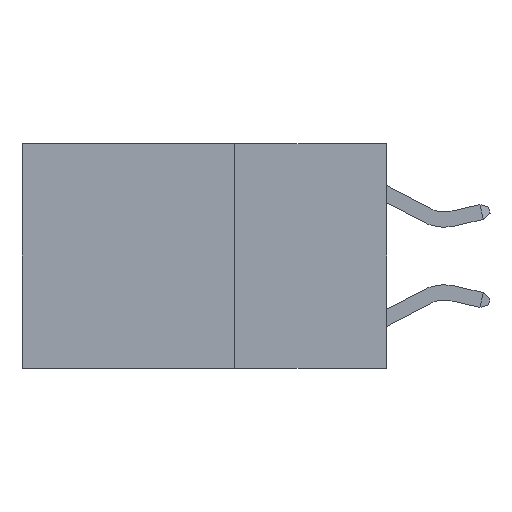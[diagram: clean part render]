
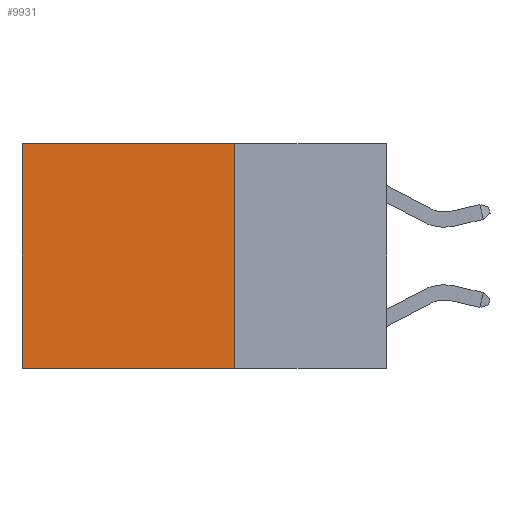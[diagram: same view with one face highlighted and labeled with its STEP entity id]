
A CAD part, left-side view. The second image highlights one B-rep face of the part: STEP entity #9931.
In plain terms, the highlighted planar face has unit normal (-1, 0, 0).
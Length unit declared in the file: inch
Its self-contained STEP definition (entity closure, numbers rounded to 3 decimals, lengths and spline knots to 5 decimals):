
#650 = VERTEX_POINT ( 'NONE', #3282 ) ;
#658 = CARTESIAN_POINT ( 'NONE',  ( 0.2625, 0.25, 0. ) ) ;
#1146 = CARTESIAN_POINT ( 'NONE',  ( 0.2625, 0.6, 0. ) ) ;
#1256 = VECTOR ( 'NONE', #19972, 39.37008 ) ;
#2601 = ORIENTED_EDGE ( 'NONE', *, *, #5508, .F. ) ;
#3282 = CARTESIAN_POINT ( 'NONE',  ( 0.2625, 0.25, 0. ) ) ;
#3354 = VERTEX_POINT ( 'NONE', #8231 ) ;
#3505 = LINE ( 'NONE', #1146, #19360 ) ;
#4098 = VERTEX_POINT ( 'NONE', #19634 ) ;
#4163 = LINE ( 'NONE', #14296, #15892 ) ;
#4839 = EDGE_CURVE ( 'NONE', #650, #3354, #13999, .T. ) ;
#5508 = EDGE_CURVE ( 'NONE', #3354, #4098, #4163, .T. ) ;
#5686 = AXIS2_PLACEMENT_3D ( 'NONE', #16736, #7236, #18332 ) ;
#6070 = VECTOR ( 'NONE', #18127, 39.37008 ) ;
#7236 = DIRECTION ( 'NONE',  ( 1., 0., 0. ) ) ;
#8231 = CARTESIAN_POINT ( 'NONE',  ( 0.2625, 0.25, -0.37 ) ) ;
#8804 = PLANE ( 'NONE',  #5686 ) ;
#8998 = FACE_OUTER_BOUND ( 'NONE', #12651, .T. ) ;
#9709 = ORIENTED_EDGE ( 'NONE', *, *, #16619, .T. ) ;
#9931 = ADVANCED_FACE ( 'NONE', ( #8998 ), #8804, .F. ) ;
#10456 = CARTESIAN_POINT ( 'NONE',  ( 0.2625, 0.6, 0. ) ) ;
#12217 = CARTESIAN_POINT ( 'NONE',  ( 0.2625, 0.25, 0. ) ) ;
#12651 = EDGE_LOOP ( 'NONE', ( #9709, #2601, #17340, #14779 ) ) ;
#12815 = VERTEX_POINT ( 'NONE', #10456 ) ;
#13999 = LINE ( 'NONE', #12217, #1256 ) ;
#14296 = CARTESIAN_POINT ( 'NONE',  ( 0.2625, 0.25, -0.37 ) ) ;
#14313 = EDGE_CURVE ( 'NONE', #650, #12815, #14587, .T. ) ;
#14587 = LINE ( 'NONE', #658, #6070 ) ;
#14779 = ORIENTED_EDGE ( 'NONE', *, *, #14313, .T. ) ;
#15847 = DIRECTION ( 'NONE',  ( 0., 1., 0. ) ) ;
#15892 = VECTOR ( 'NONE', #15847, 39.37008 ) ;
#16619 = EDGE_CURVE ( 'NONE', #12815, #4098, #3505, .T. ) ;
#16736 = CARTESIAN_POINT ( 'NONE',  ( 0.2625, 0.25, 0. ) ) ;
#16937 = DIRECTION ( 'NONE',  ( 0., 0., -1. ) ) ;
#17340 = ORIENTED_EDGE ( 'NONE', *, *, #4839, .F. ) ;
#18127 = DIRECTION ( 'NONE',  ( 0., 1., 0. ) ) ;
#18332 = DIRECTION ( 'NONE',  ( 0., 0., -1. ) ) ;
#19360 = VECTOR ( 'NONE', #16937, 39.37008 ) ;
#19634 = CARTESIAN_POINT ( 'NONE',  ( 0.2625, 0.6, -0.37 ) ) ;
#19972 = DIRECTION ( 'NONE',  ( 0., 0., -1. ) ) ;
